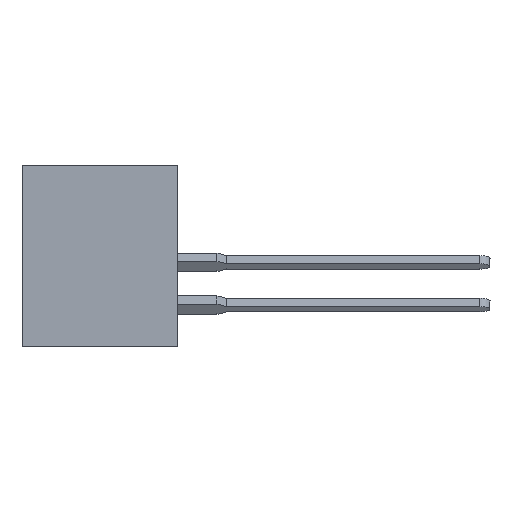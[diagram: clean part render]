
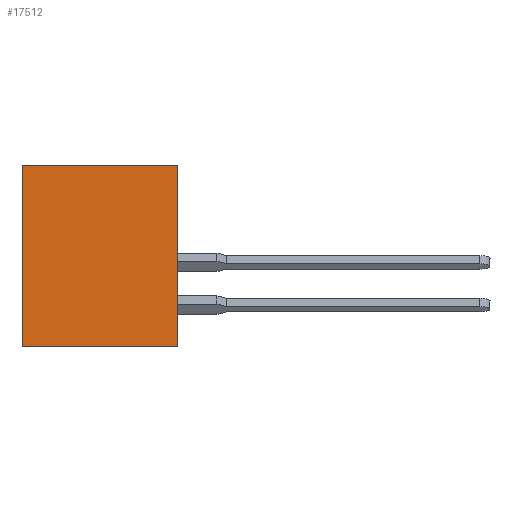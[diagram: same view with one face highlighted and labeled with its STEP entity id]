
A CAD part, left-side view. The second image highlights one B-rep face of the part: STEP entity #17512.
In plain terms, the highlighted planar face has unit normal (-1, 0, 0).
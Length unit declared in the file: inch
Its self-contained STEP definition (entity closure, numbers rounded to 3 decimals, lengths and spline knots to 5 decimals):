
#380 = DIRECTION ( 'NONE',  ( 1., 0., 0. ) ) ;
#633 = CARTESIAN_POINT ( 'NONE',  ( 0., 0., 0. ) ) ;
#735 = ORIENTED_EDGE ( 'NONE', *, *, #8830, .F. ) ;
#1108 = CARTESIAN_POINT ( 'NONE',  ( 0., 0.453, -0.531 ) ) ;
#2928 = CARTESIAN_POINT ( 'NONE',  ( 0., 0.453, 0. ) ) ;
#4924 = DIRECTION ( 'NONE',  ( 0., -1., 0. ) ) ;
#4932 = DIRECTION ( 'NONE',  ( 0., -1., 0. ) ) ;
#4996 = CARTESIAN_POINT ( 'NONE',  ( 0., 0.453, -0.531 ) ) ;
#7063 = CARTESIAN_POINT ( 'NONE',  ( 0., 0., -0.531 ) ) ;
#8691 = CARTESIAN_POINT ( 'NONE',  ( 0., 0.453, 0. ) ) ;
#8830 = EDGE_CURVE ( 'NONE', #21447, #14565, #12834, .T. ) ;
#10087 = FACE_OUTER_BOUND ( 'NONE', #21221, .T. ) ;
#10734 = DIRECTION ( 'NONE',  ( 0., 0., -1. ) ) ;
#11799 = VECTOR ( 'NONE', #4924, 39.37008 ) ;
#12467 = LINE ( 'NONE', #1108, #20577 ) ;
#12482 = DIRECTION ( 'NONE',  ( 0., 0., 1. ) ) ;
#12588 = PLANE ( 'NONE',  #19927 ) ;
#12834 = LINE ( 'NONE', #8691, #21763 ) ;
#12843 = DIRECTION ( 'NONE',  ( 0., 0., 1. ) ) ;
#13308 = ORIENTED_EDGE ( 'NONE', *, *, #17084, .T. ) ;
#13334 = ORIENTED_EDGE ( 'NONE', *, *, #20617, .F. ) ;
#14268 = LINE ( 'NONE', #633, #19632 ) ;
#14565 = VERTEX_POINT ( 'NONE', #21344 ) ;
#14723 = EDGE_CURVE ( 'NONE', #21447, #18672, #12467, .T. ) ;
#15093 = CARTESIAN_POINT ( 'NONE',  ( 0., 0., 0. ) ) ;
#17084 = EDGE_CURVE ( 'NONE', #18672, #19084, #14268, .T. ) ;
#17512 = ADVANCED_FACE ( 'NONE', ( #10087 ), #12588, .F. ) ;
#17905 = CARTESIAN_POINT ( 'NONE',  ( 0., 0.453, 0. ) ) ;
#18192 = ORIENTED_EDGE ( 'NONE', *, *, #14723, .T. ) ;
#18672 = VERTEX_POINT ( 'NONE', #7063 ) ;
#19084 = VERTEX_POINT ( 'NONE', #15093 ) ;
#19632 = VECTOR ( 'NONE', #12843, 39.37008 ) ;
#19927 = AXIS2_PLACEMENT_3D ( 'NONE', #17905, #380, #10734 ) ;
#20577 = VECTOR ( 'NONE', #4932, 39.37008 ) ;
#20617 = EDGE_CURVE ( 'NONE', #14565, #19084, #20762, .T. ) ;
#20762 = LINE ( 'NONE', #2928, #11799 ) ;
#21221 = EDGE_LOOP ( 'NONE', ( #13308, #13334, #735, #18192 ) ) ;
#21344 = CARTESIAN_POINT ( 'NONE',  ( 0., 0.453, 0. ) ) ;
#21447 = VERTEX_POINT ( 'NONE', #4996 ) ;
#21763 = VECTOR ( 'NONE', #12482, 39.37008 ) ;
